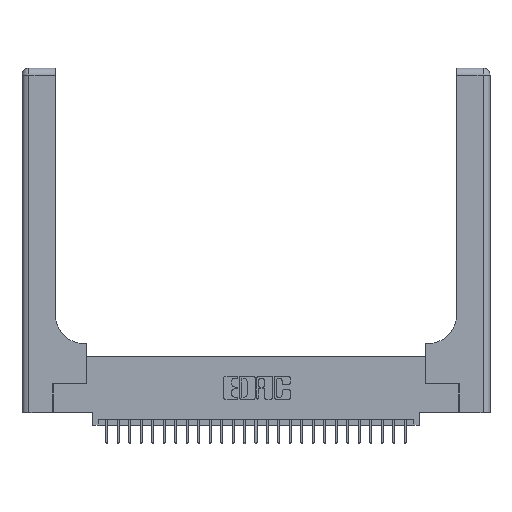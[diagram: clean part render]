
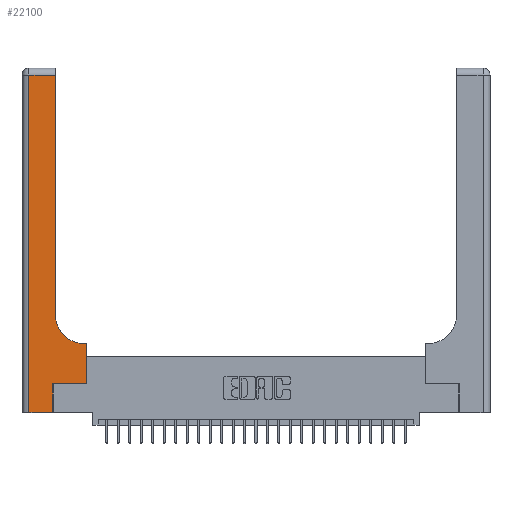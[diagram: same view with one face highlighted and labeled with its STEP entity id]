
A CAD part, top view. The second image highlights one B-rep face of the part: STEP entity #22100.
In plain terms, the highlighted planar face has unit normal (0, 0, 1).
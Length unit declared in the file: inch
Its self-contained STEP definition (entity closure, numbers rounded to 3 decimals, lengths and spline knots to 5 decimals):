
#200 = CARTESIAN_POINT ( 'NONE',  ( 0.2915, 2.94, 0.37 ) ) ;
#263 = DIRECTION ( 'NONE',  ( 1., 0., 0. ) ) ;
#412 = LINE ( 'NONE', #22760, #15918 ) ;
#1263 = EDGE_CURVE ( 'NONE', #19544, #8088, #4223, .T. ) ;
#1830 = DIRECTION ( 'NONE',  ( 0., 0., -1. ) ) ;
#2480 = CARTESIAN_POINT ( 'NONE',  ( 0.5585, 0.6, 0.37 ) ) ;
#2883 = EDGE_CURVE ( 'NONE', #24223, #23573, #7582, .T. ) ;
#2940 = DIRECTION ( 'NONE',  ( -1., 0., 0. ) ) ;
#3393 = VECTOR ( 'NONE', #19239, 39.37008 ) ;
#4122 = DIRECTION ( 'NONE',  ( 0., 0., -1. ) ) ;
#4223 = LINE ( 'NONE', #24865, #27049 ) ;
#5220 = ORIENTED_EDGE ( 'NONE', *, *, #7275, .T. ) ;
#5559 = ORIENTED_EDGE ( 'NONE', *, *, #28604, .T. ) ;
#5600 = VERTEX_POINT ( 'NONE', #18588 ) ;
#5726 = VERTEX_POINT ( 'NONE', #18972 ) ;
#6111 = CARTESIAN_POINT ( 'NONE',  ( 0.06, 3., 0.37 ) ) ;
#7114 = EDGE_LOOP ( 'NONE', ( #17606, #27004, #15886, #5559, #20793, #16254, #5220, #9053, #21512 ) ) ;
#7275 = EDGE_CURVE ( 'NONE', #22076, #19544, #15976, .T. ) ;
#7536 = CARTESIAN_POINT ( 'NONE',  ( 0., 0., 0.37 ) ) ;
#7582 = LINE ( 'NONE', #8521, #18635 ) ;
#8088 = VERTEX_POINT ( 'NONE', #12949 ) ;
#8303 = LINE ( 'NONE', #26752, #19372 ) ;
#8324 = DIRECTION ( 'NONE',  ( 0., -1., 0. ) ) ;
#8377 = AXIS2_PLACEMENT_3D ( 'NONE', #17318, #4122, #19583 ) ;
#8521 = CARTESIAN_POINT ( 'NONE',  ( 0.2915, 3., 0.37 ) ) ;
#8811 = LINE ( 'NONE', #7536, #26468 ) ;
#9053 = ORIENTED_EDGE ( 'NONE', *, *, #1263, .T. ) ;
#9479 = EDGE_CURVE ( 'NONE', #8088, #24223, #21543, .T. ) ;
#9664 = DIRECTION ( 'NONE',  ( 1., 0., 0. ) ) ;
#11334 = LINE ( 'NONE', #6111, #17204 ) ;
#12779 = PLANE ( 'NONE',  #19146 ) ;
#12949 = CARTESIAN_POINT ( 'NONE',  ( 0.5415, 0.6, 0.37 ) ) ;
#14728 = CARTESIAN_POINT ( 'NONE',  ( 0.06, 0., 0.37 ) ) ;
#15886 = ORIENTED_EDGE ( 'NONE', *, *, #20583, .T. ) ;
#15918 = VECTOR ( 'NONE', #2940, 39.37008 ) ;
#15976 = LINE ( 'NONE', #28121, #27088 ) ;
#16214 = FACE_OUTER_BOUND ( 'NONE', #7114, .T. ) ;
#16254 = ORIENTED_EDGE ( 'NONE', *, *, #19535, .T. ) ;
#16814 = CARTESIAN_POINT ( 'NONE',  ( 0.06, 2.94, 0.37 ) ) ;
#17204 = VECTOR ( 'NONE', #8324, 39.37008 ) ;
#17230 = DIRECTION ( 'NONE',  ( -1., 0., 0. ) ) ;
#17284 = DIRECTION ( 'NONE',  ( 0., 1., 0. ) ) ;
#17318 = CARTESIAN_POINT ( 'NONE',  ( 0.5415, 0.85, 0.37 ) ) ;
#17606 = ORIENTED_EDGE ( 'NONE', *, *, #2883, .T. ) ;
#18588 = CARTESIAN_POINT ( 'NONE',  ( 0.269, 0., 0.37 ) ) ;
#18635 = VECTOR ( 'NONE', #17284, 39.37008 ) ;
#18972 = CARTESIAN_POINT ( 'NONE',  ( 0.269, 0.25, 0.37 ) ) ;
#19146 = AXIS2_PLACEMENT_3D ( 'NONE', #28280, #1830, #17230 ) ;
#19239 = DIRECTION ( 'NONE',  ( 0., 1., 0. ) ) ;
#19372 = VECTOR ( 'NONE', #263, 39.37008 ) ;
#19395 = CARTESIAN_POINT ( 'NONE',  ( 0.5585, 0.25, 0.37 ) ) ;
#19535 = EDGE_CURVE ( 'NONE', #5726, #22076, #8303, .T. ) ;
#19544 = VERTEX_POINT ( 'NONE', #2480 ) ;
#19583 = DIRECTION ( 'NONE',  ( 1., 0., 0. ) ) ;
#20583 = EDGE_CURVE ( 'NONE', #25864, #27043, #11334, .T. ) ;
#20793 = ORIENTED_EDGE ( 'NONE', *, *, #23293, .T. ) ;
#21512 = ORIENTED_EDGE ( 'NONE', *, *, #9479, .T. ) ;
#21543 = CIRCLE ( 'NONE', #8377, 0.25 ) ;
#22076 = VERTEX_POINT ( 'NONE', #19395 ) ;
#22100 = ADVANCED_FACE ( 'NONE', ( #16214 ), #12779, .F. ) ;
#22760 = CARTESIAN_POINT ( 'NONE',  ( 0., 2.94, 0.37 ) ) ;
#23293 = EDGE_CURVE ( 'NONE', #5600, #5726, #26913, .T. ) ;
#23573 = VERTEX_POINT ( 'NONE', #200 ) ;
#23916 = CARTESIAN_POINT ( 'NONE',  ( 0.2915, 0.85, 0.37 ) ) ;
#24223 = VERTEX_POINT ( 'NONE', #23916 ) ;
#24865 = CARTESIAN_POINT ( 'NONE',  ( 0.2915, 0.6, 0.37 ) ) ;
#25837 = CARTESIAN_POINT ( 'NONE',  ( 0.269, 0., 0.37 ) ) ;
#25864 = VERTEX_POINT ( 'NONE', #16814 ) ;
#26018 = DIRECTION ( 'NONE',  ( 0., 1., 0. ) ) ;
#26468 = VECTOR ( 'NONE', #9664, 39.37008 ) ;
#26752 = CARTESIAN_POINT ( 'NONE',  ( 0.269, 0.25, 0.37 ) ) ;
#26913 = LINE ( 'NONE', #25837, #3393 ) ;
#27004 = ORIENTED_EDGE ( 'NONE', *, *, #27985, .T. ) ;
#27043 = VERTEX_POINT ( 'NONE', #14728 ) ;
#27049 = VECTOR ( 'NONE', #27065, 39.37008 ) ;
#27065 = DIRECTION ( 'NONE',  ( -1., 0., 0. ) ) ;
#27088 = VECTOR ( 'NONE', #26018, 39.37008 ) ;
#27985 = EDGE_CURVE ( 'NONE', #23573, #25864, #412, .T. ) ;
#28121 = CARTESIAN_POINT ( 'NONE',  ( 0.5585, 0.25, 0.37 ) ) ;
#28280 = CARTESIAN_POINT ( 'NONE',  ( 0., 3., 0.37 ) ) ;
#28604 = EDGE_CURVE ( 'NONE', #27043, #5600, #8811, .T. ) ;
